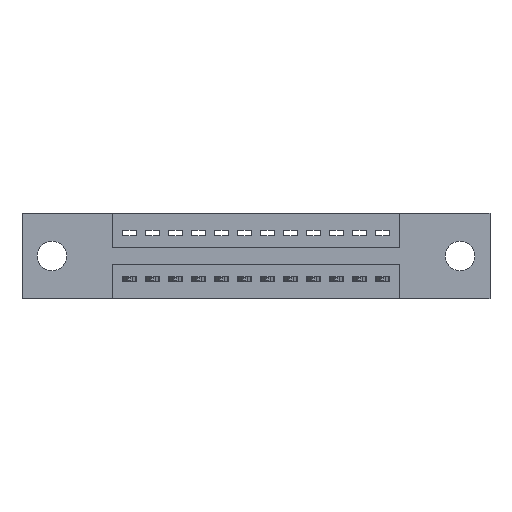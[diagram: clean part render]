
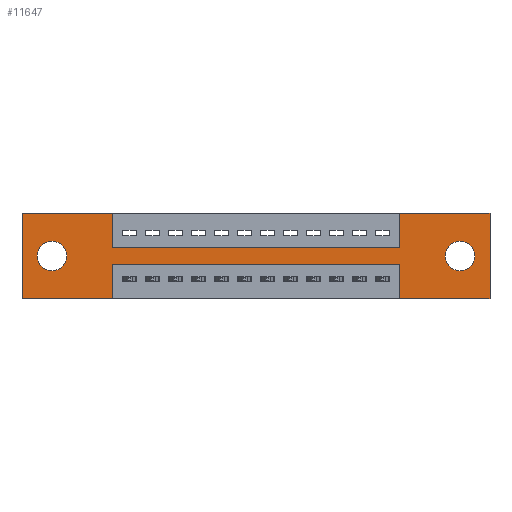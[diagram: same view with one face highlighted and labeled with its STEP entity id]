
A CAD part, front view. The second image highlights one B-rep face of the part: STEP entity #11647.
In plain terms, the highlighted planar face has unit normal (0, -1, 0).
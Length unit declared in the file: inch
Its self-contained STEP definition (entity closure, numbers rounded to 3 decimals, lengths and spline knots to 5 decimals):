
#6 = EDGE_CURVE ( 'NONE', #3559, #11109, #10848, .T. ) ;
#15 = VERTEX_POINT ( 'NONE', #8235 ) ;
#147 = VECTOR ( 'NONE', #4198, 39.37008 ) ;
#173 = CARTESIAN_POINT ( 'NONE',  ( 0., 0., -0.37 ) ) ;
#408 = ORIENTED_EDGE ( 'NONE', *, *, #9210, .F. ) ;
#586 = LINE ( 'NONE', #2318, #10673 ) ;
#792 = DIRECTION ( 'NONE',  ( 1., 0., 0. ) ) ;
#833 = EDGE_LOOP ( 'NONE', ( #12816, #1535 ) ) ;
#915 = VECTOR ( 'NONE', #2167, 39.37008 ) ;
#1011 = LINE ( 'NONE', #10121, #9364 ) ;
#1023 = ORIENTED_EDGE ( 'NONE', *, *, #3528, .F. ) ;
#1319 = ORIENTED_EDGE ( 'NONE', *, *, #3354, .F. ) ;
#1512 = VECTOR ( 'NONE', #10820, 39.37008 ) ;
#1535 = ORIENTED_EDGE ( 'NONE', *, *, #7567, .T. ) ;
#1769 = EDGE_CURVE ( 'NONE', #15, #11784, #9368, .T. ) ;
#2051 = DIRECTION ( 'NONE',  ( 0., 0., -1. ) ) ;
#2167 = DIRECTION ( 'NONE',  ( 0., 0., -1. ) ) ;
#2189 = CARTESIAN_POINT ( 'NONE',  ( 0.3925, 0., -0.22 ) ) ;
#2196 = DIRECTION ( 'NONE',  ( 0., -1., 0. ) ) ;
#2257 = VERTEX_POINT ( 'NONE', #5162 ) ;
#2318 = CARTESIAN_POINT ( 'NONE',  ( 0., 0., -0.37 ) ) ;
#2360 = VERTEX_POINT ( 'NONE', #8217 ) ;
#2502 = CARTESIAN_POINT ( 'NONE',  ( 0.3925, 0., -0.37 ) ) ;
#2619 = FACE_BOUND ( 'NONE', #6417, .T. ) ;
#2657 = AXIS2_PLACEMENT_3D ( 'NONE', #4811, #10183, #5879 ) ;
#2749 = CARTESIAN_POINT ( 'NONE',  ( 1.905, 0., -0.121 ) ) ;
#2907 = CARTESIAN_POINT ( 'NONE',  ( 0.3925, 0., -0.15 ) ) ;
#3145 = VERTEX_POINT ( 'NONE', #7803 ) ;
#3232 = CARTESIAN_POINT ( 'NONE',  ( 0., 0., 0. ) ) ;
#3273 = DIRECTION ( 'NONE',  ( 0., 1., 0. ) ) ;
#3300 = DIRECTION ( 'NONE',  ( -1., 0., 0. ) ) ;
#3354 = EDGE_CURVE ( 'NONE', #11784, #10995, #6946, .T. ) ;
#3422 = CIRCLE ( 'NONE', #8783, 0.064 ) ;
#3528 = EDGE_CURVE ( 'NONE', #10995, #6882, #4249, .T. ) ;
#3559 = VERTEX_POINT ( 'NONE', #12437 ) ;
#3714 = ORIENTED_EDGE ( 'NONE', *, *, #4704, .T. ) ;
#3767 = EDGE_CURVE ( 'NONE', #12961, #4794, #9815, .T. ) ;
#3943 = CARTESIAN_POINT ( 'NONE',  ( 0., 0., 0. ) ) ;
#4092 = DIRECTION ( 'NONE',  ( 0., 0., 1. ) ) ;
#4197 = DIRECTION ( 'NONE',  ( 0., 0., -1. ) ) ;
#4198 = DIRECTION ( 'NONE',  ( 1., 0., 0. ) ) ;
#4249 = LINE ( 'NONE', #6155, #11369 ) ;
#4427 = LINE ( 'NONE', #7933, #6133 ) ;
#4555 = CARTESIAN_POINT ( 'NONE',  ( 0.3925, 0., -0.22 ) ) ;
#4556 = VERTEX_POINT ( 'NONE', #2502 ) ;
#4619 = EDGE_CURVE ( 'NONE', #3145, #12961, #9546, .T. ) ;
#4647 = CIRCLE ( 'NONE', #5951, 0.064 ) ;
#4698 = VECTOR ( 'NONE', #792, 39.37008 ) ;
#4704 = EDGE_CURVE ( 'NONE', #2360, #6738, #7822, .T. ) ;
#4725 = CARTESIAN_POINT ( 'NONE',  ( 0., 0., 0. ) ) ;
#4740 = DIRECTION ( 'NONE',  ( 0., 0., 1. ) ) ;
#4762 = FACE_OUTER_BOUND ( 'NONE', #9126, .T. ) ;
#4794 = VERTEX_POINT ( 'NONE', #2189 ) ;
#4811 = CARTESIAN_POINT ( 'NONE',  ( 0.13, 0., -0.185 ) ) ;
#4856 = DIRECTION ( 'NONE',  ( 0., 0., -1. ) ) ;
#5081 = FACE_BOUND ( 'NONE', #833, .T. ) ;
#5141 = PLANE ( 'NONE',  #6767 ) ;
#5162 = CARTESIAN_POINT ( 'NONE',  ( 1.905, 0., -0.249 ) ) ;
#5663 = CARTESIAN_POINT ( 'NONE',  ( 1.905, 0., -0.185 ) ) ;
#5839 = ORIENTED_EDGE ( 'NONE', *, *, #9567, .F. ) ;
#5879 = DIRECTION ( 'NONE',  ( 0., 0., 1. ) ) ;
#5951 = AXIS2_PLACEMENT_3D ( 'NONE', #9312, #3273, #4197 ) ;
#5957 = ORIENTED_EDGE ( 'NONE', *, *, #3767, .F. ) ;
#6133 = VECTOR ( 'NONE', #4740, 39.37008 ) ;
#6155 = CARTESIAN_POINT ( 'NONE',  ( 0.3925, 0., 0. ) ) ;
#6417 = EDGE_LOOP ( 'NONE', ( #10872, #3714 ) ) ;
#6607 = EDGE_CURVE ( 'NONE', #7505, #3559, #4427, .T. ) ;
#6727 = CARTESIAN_POINT ( 'NONE',  ( 1.6425, 0., -0.15 ) ) ;
#6738 = VERTEX_POINT ( 'NONE', #11983 ) ;
#6749 = CARTESIAN_POINT ( 'NONE',  ( 0., 0., 0. ) ) ;
#6767 = AXIS2_PLACEMENT_3D ( 'NONE', #173, #2196, #7187 ) ;
#6882 = VERTEX_POINT ( 'NONE', #11270 ) ;
#6946 = LINE ( 'NONE', #4725, #4698 ) ;
#7163 = AXIS2_PLACEMENT_3D ( 'NONE', #5663, #12799, #4856 ) ;
#7187 = DIRECTION ( 'NONE',  ( 0., 0., -1. ) ) ;
#7420 = LINE ( 'NONE', #12246, #915 ) ;
#7460 = CIRCLE ( 'NONE', #7163, 0.064 ) ;
#7505 = VERTEX_POINT ( 'NONE', #6727 ) ;
#7531 = VERTEX_POINT ( 'NONE', #2749 ) ;
#7567 = EDGE_CURVE ( 'NONE', #2257, #7531, #7460, .T. ) ;
#7803 = CARTESIAN_POINT ( 'NONE',  ( 1.6425, 0., -0.37 ) ) ;
#7822 = CIRCLE ( 'NONE', #2657, 0.064 ) ;
#7933 = CARTESIAN_POINT ( 'NONE',  ( 1.6425, 0., 0. ) ) ;
#7972 = VECTOR ( 'NONE', #11703, 39.37008 ) ;
#7974 = VERTEX_POINT ( 'NONE', #8708 ) ;
#8141 = DIRECTION ( 'NONE',  ( 0., 1., 0. ) ) ;
#8173 = EDGE_CURVE ( 'NONE', #11109, #7974, #1011, .T. ) ;
#8196 = DIRECTION ( 'NONE',  ( -1., 0., 0. ) ) ;
#8217 = CARTESIAN_POINT ( 'NONE',  ( 0.13, 0., -0.249 ) ) ;
#8235 = CARTESIAN_POINT ( 'NONE',  ( 0., 0., -0.37 ) ) ;
#8273 = ORIENTED_EDGE ( 'NONE', *, *, #11654, .F. ) ;
#8408 = EDGE_CURVE ( 'NONE', #4794, #4556, #7420, .T. ) ;
#8708 = CARTESIAN_POINT ( 'NONE',  ( 2.035, 0., -0.37 ) ) ;
#8783 = AXIS2_PLACEMENT_3D ( 'NONE', #10171, #8141, #4092 ) ;
#8953 = CARTESIAN_POINT ( 'NONE',  ( 0.3925, 0., 0. ) ) ;
#8958 = EDGE_CURVE ( 'NONE', #6738, #2360, #3422, .T. ) ;
#9126 = EDGE_LOOP ( 'NONE', ( #11493, #5957, #12506, #8273, #10122, #11608, #11447, #408, #1023, #1319, #13040, #5839 ) ) ;
#9210 = EDGE_CURVE ( 'NONE', #6882, #7505, #11508, .T. ) ;
#9312 = CARTESIAN_POINT ( 'NONE',  ( 1.905, 0., -0.185 ) ) ;
#9364 = VECTOR ( 'NONE', #2051, 39.37008 ) ;
#9368 = LINE ( 'NONE', #6749, #7972 ) ;
#9546 = LINE ( 'NONE', #11517, #1512 ) ;
#9567 = EDGE_CURVE ( 'NONE', #4556, #15, #586, .T. ) ;
#9815 = LINE ( 'NONE', #4555, #11112 ) ;
#9872 = EDGE_CURVE ( 'NONE', #7531, #2257, #4647, .T. ) ;
#9990 = VECTOR ( 'NONE', #8196, 39.37008 ) ;
#10121 = CARTESIAN_POINT ( 'NONE',  ( 2.035, 0., 0. ) ) ;
#10122 = ORIENTED_EDGE ( 'NONE', *, *, #8173, .F. ) ;
#10140 = CARTESIAN_POINT ( 'NONE',  ( 0., 0., -0.37 ) ) ;
#10171 = CARTESIAN_POINT ( 'NONE',  ( 0.13, 0., -0.185 ) ) ;
#10183 = DIRECTION ( 'NONE',  ( 0., 1., 0. ) ) ;
#10673 = VECTOR ( 'NONE', #3300, 39.37008 ) ;
#10820 = DIRECTION ( 'NONE',  ( 0., 0., 1. ) ) ;
#10848 = LINE ( 'NONE', #3232, #147 ) ;
#10872 = ORIENTED_EDGE ( 'NONE', *, *, #8958, .T. ) ;
#10995 = VERTEX_POINT ( 'NONE', #8953 ) ;
#11109 = VERTEX_POINT ( 'NONE', #11145 ) ;
#11112 = VECTOR ( 'NONE', #12562, 39.37008 ) ;
#11145 = CARTESIAN_POINT ( 'NONE',  ( 2.035, 0., 0. ) ) ;
#11270 = CARTESIAN_POINT ( 'NONE',  ( 0.3925, 0., -0.15 ) ) ;
#11369 = VECTOR ( 'NONE', #12116, 39.37008 ) ;
#11447 = ORIENTED_EDGE ( 'NONE', *, *, #6607, .F. ) ;
#11493 = ORIENTED_EDGE ( 'NONE', *, *, #8408, .F. ) ;
#11508 = LINE ( 'NONE', #2907, #12091 ) ;
#11517 = CARTESIAN_POINT ( 'NONE',  ( 1.6425, 0., -0.37 ) ) ;
#11608 = ORIENTED_EDGE ( 'NONE', *, *, #6, .F. ) ;
#11647 = ADVANCED_FACE ( 'NONE', ( #5081, #2619, #4762 ), #5141, .T. ) ;
#11654 = EDGE_CURVE ( 'NONE', #7974, #3145, #13056, .T. ) ;
#11703 = DIRECTION ( 'NONE',  ( 0., 0., 1. ) ) ;
#11784 = VERTEX_POINT ( 'NONE', #3943 ) ;
#11926 = DIRECTION ( 'NONE',  ( 1., 0., 0. ) ) ;
#11983 = CARTESIAN_POINT ( 'NONE',  ( 0.13, 0., -0.121 ) ) ;
#12091 = VECTOR ( 'NONE', #11926, 39.37008 ) ;
#12116 = DIRECTION ( 'NONE',  ( 0., 0., -1. ) ) ;
#12156 = CARTESIAN_POINT ( 'NONE',  ( 1.6425, 0., -0.22 ) ) ;
#12246 = CARTESIAN_POINT ( 'NONE',  ( 0.3925, 0., -0.37 ) ) ;
#12437 = CARTESIAN_POINT ( 'NONE',  ( 1.6425, 0., 0. ) ) ;
#12506 = ORIENTED_EDGE ( 'NONE', *, *, #4619, .F. ) ;
#12562 = DIRECTION ( 'NONE',  ( -1., 0., 0. ) ) ;
#12799 = DIRECTION ( 'NONE',  ( 0., 1., 0. ) ) ;
#12816 = ORIENTED_EDGE ( 'NONE', *, *, #9872, .T. ) ;
#12961 = VERTEX_POINT ( 'NONE', #12156 ) ;
#13040 = ORIENTED_EDGE ( 'NONE', *, *, #1769, .F. ) ;
#13056 = LINE ( 'NONE', #10140, #9990 ) ;
